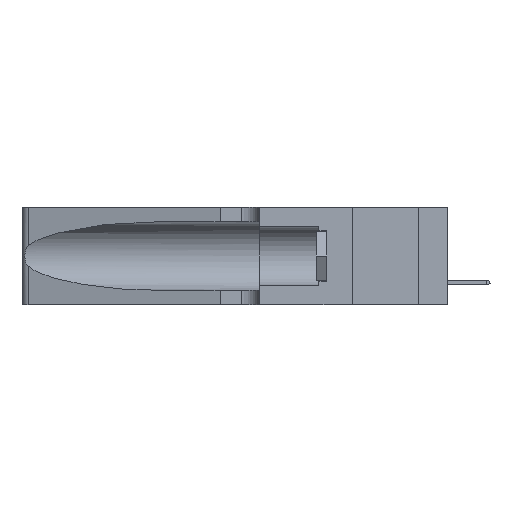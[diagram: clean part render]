
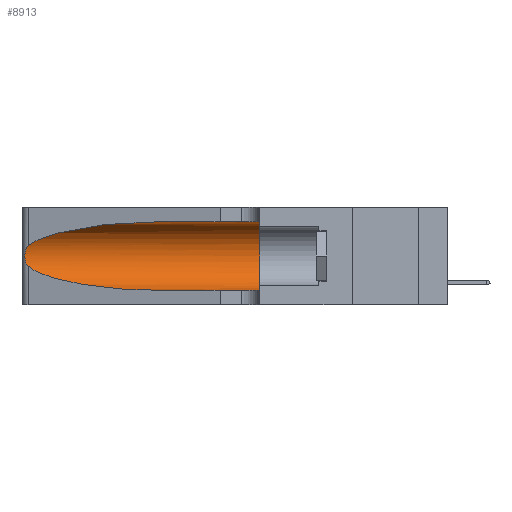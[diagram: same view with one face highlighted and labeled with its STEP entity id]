
A CAD part, left-side view. The second image highlights one B-rep face of the part: STEP entity #8913.
In plain terms, the highlighted cylindrical face has radius 3.308 mm (diameter 6.617 mm), a partial arc.
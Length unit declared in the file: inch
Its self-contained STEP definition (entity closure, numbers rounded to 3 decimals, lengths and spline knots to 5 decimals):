
#789 = CARTESIAN_POINT ( 'NONE',  ( 0.1305, 0.35, 0.05475 ) ) ;
#1953 = B_SPLINE_CURVE_WITH_KNOTS ( 'NONE', 3,
 ( #25652, #28455, #9611, #30937, #12276, #33630, #25879, #31040, #31159, #15073, #20415, #17869, #9949, #28571 ),
 .UNSPECIFIED., .F., .F.,
 ( 4, 2, 2, 2, 2, 2, 4 ),
 ( 0., 0.00027, 0.00053, 0.00107, 0.0016, 0.00187, 0.00214 ),
 .UNSPECIFIED. ) ;
#3556 = CARTESIAN_POINT ( 'NONE',  ( 0.18966, 0.96281, 0.05475 ) ) ;
#3749 = ORIENTED_EDGE ( 'NONE', *, *, #12329, .T. ) ;
#3765 = FACE_OUTER_BOUND ( 'NONE', #19042, .T. ) ;
#4085 = CIRCLE ( 'NONE', #7593, 0.13025 ) ;
#4809 = CARTESIAN_POINT ( 'NONE',  ( 0.2373, 1.15595, 0.28018 ) ) ;
#4878 = LINE ( 'NONE', #30529, #29453 ) ;
#5195 = DIRECTION ( 'NONE',  ( 0., -1., 0. ) ) ;
#5419 = EDGE_CURVE ( 'NONE', #30659, #13672, #1953, .T. ) ;
#6132 = CARTESIAN_POINT ( 'NONE',  ( 0.1305, 1.61858, 0.185 ) ) ;
#6133 = DIRECTION ( 'NONE',  ( 0., 1., 0. ) ) ;
#7593 = AXIS2_PLACEMENT_3D ( 'NONE', #32778, #6133, #11466 ) ;
#8037 = CARTESIAN_POINT ( 'NONE',  ( 0.1305, 0.72297, 0.05475 ) ) ;
#8913 = ADVANCED_FACE ( 'NONE', ( #3765 ), #20054, .F. ) ;
#9611 = CARTESIAN_POINT ( 'NONE',  ( 0.25639, 1.23184, 0.21858 ) ) ;
#9949 = CARTESIAN_POINT ( 'NONE',  ( 0.25555, 1.22993, 0.14849 ) ) ;
#11466 = DIRECTION ( 'NONE',  ( 0., 0., 1. ) ) ;
#11653 = CARTESIAN_POINT ( 'NONE',  ( 0.25487, 1.22718, 0.22369 ) ) ;
#12276 = CARTESIAN_POINT ( 'NONE',  ( 0.25854, 1.2359, 0.20912 ) ) ;
#12329 = EDGE_CURVE ( 'NONE', #13206, #30659, #30320, .T. ) ;
#13206 = VERTEX_POINT ( 'NONE', #31715 ) ;
#13304 = AXIS2_PLACEMENT_3D ( 'NONE', #6132, #24704, #30208 ) ;
#13672 = VERTEX_POINT ( 'NONE', #20605 ) ;
#13764 = ORIENTED_EDGE ( 'NONE', *, *, #5419, .T. ) ;
#14542 = VECTOR ( 'NONE', #5195, 39.37008 ) ;
#15073 = CARTESIAN_POINT ( 'NONE',  ( 0.25856, 1.23593, 0.16098 ) ) ;
#15747 = CARTESIAN_POINT ( 'NONE',  ( 0.25487, 1.22718, 0.22369 ) ) ;
#17377 = ORIENTED_EDGE ( 'NONE', *, *, #22622, .F. ) ;
#17453 = ORIENTED_EDGE ( 'NONE', *, *, #29007, .F. ) ;
#17869 = CARTESIAN_POINT ( 'NONE',  ( 0.25639, 1.23186, 0.15144 ) ) ;
#18022 = ORIENTED_EDGE ( 'NONE', *, *, #28373, .T. ) ;
#18400 = CARTESIAN_POINT ( 'NONE',  ( 0.18966, 0.96281, 0.31525 ) ) ;
#18597 = CARTESIAN_POINT ( 'NONE',  ( 0.2373, 1.15595, 0.08982 ) ) ;
#18759 = VERTEX_POINT ( 'NONE', #8037 ) ;
#19042 = EDGE_LOOP ( 'NONE', ( #3749, #13764, #18022, #25834, #17453, #17377 ) ) ;
#19198 = CARTESIAN_POINT ( 'NONE',  ( 0.25487, 1.22718, 0.14631 ) ) ;
#20054 = CYLINDRICAL_SURFACE ( 'NONE', #13304, 0.13025 ) ;
#20055 = DIRECTION ( 'NONE',  ( 0., -1., 0. ) ) ;
#20415 = CARTESIAN_POINT ( 'NONE',  ( 0.25789, 1.23486, 0.15765 ) ) ;
#20605 = CARTESIAN_POINT ( 'NONE',  ( 0.25487, 1.22718, 0.14631 ) ) ;
#20797 = LINE ( 'NONE', #21150, #14542 ) ;
#21150 = CARTESIAN_POINT ( 'NONE',  ( 0.1305, 1.61858, 0.31525 ) ) ;
#22183 = CARTESIAN_POINT ( 'NONE',  ( 0.1305, 0.72297, 0.05475 ) ) ;
#22622 = EDGE_CURVE ( 'NONE', #13206, #25965, #20797, .T. ) ;
#23707 =( BOUNDED_CURVE ( )  B_SPLINE_CURVE ( 3, ( #19198, #18597, #3556, #22183 ),
 .UNSPECIFIED., .F., .T. ) 
 B_SPLINE_CURVE_WITH_KNOTS ( ( 4, 4 ),
 ( 3.44316, 4.71239 ),
 .UNSPECIFIED. ) 
 CURVE ( )  GEOMETRIC_REPRESENTATION_ITEM ( )  RATIONAL_B_SPLINE_CURVE ( ( 1., 0.87, 0.87, 1. ) ) 
 REPRESENTATION_ITEM ( '' )  );
#24704 = DIRECTION ( 'NONE',  ( 0., -1., 0. ) ) ;
#25652 = CARTESIAN_POINT ( 'NONE',  ( 0.25487, 1.22718, 0.22369 ) ) ;
#25834 = ORIENTED_EDGE ( 'NONE', *, *, #29304, .T. ) ;
#25879 = CARTESIAN_POINT ( 'NONE',  ( 0.26075, 1.23896, 0.19203 ) ) ;
#25965 = VERTEX_POINT ( 'NONE', #26298 ) ;
#26298 = CARTESIAN_POINT ( 'NONE',  ( 0.1305, 0.35, 0.31525 ) ) ;
#28175 = VERTEX_POINT ( 'NONE', #789 ) ;
#28373 = EDGE_CURVE ( 'NONE', #13672, #18759, #23707, .T. ) ;
#28455 = CARTESIAN_POINT ( 'NONE',  ( 0.25555, 1.22994, 0.2215 ) ) ;
#28571 = CARTESIAN_POINT ( 'NONE',  ( 0.25487, 1.22718, 0.14631 ) ) ;
#29007 = EDGE_CURVE ( 'NONE', #25965, #28175, #4085, .T. ) ;
#29304 = EDGE_CURVE ( 'NONE', #18759, #28175, #4878, .T. ) ;
#29453 = VECTOR ( 'NONE', #20055, 39.37008 ) ;
#30208 = DIRECTION ( 'NONE',  ( 0., 0., -1. ) ) ;
#30320 =( BOUNDED_CURVE ( )  B_SPLINE_CURVE ( 3, ( #31262, #18400, #4809, #15747 ),
 .UNSPECIFIED., .F., .T. ) 
 B_SPLINE_CURVE_WITH_KNOTS ( ( 4, 4 ),
 ( 1.5708, 2.84003 ),
 .UNSPECIFIED. ) 
 CURVE ( )  GEOMETRIC_REPRESENTATION_ITEM ( )  RATIONAL_B_SPLINE_CURVE ( ( 1., 0.87, 0.87, 1. ) ) 
 REPRESENTATION_ITEM ( '' )  );
#30529 = CARTESIAN_POINT ( 'NONE',  ( 0.1305, 1.61858, 0.05475 ) ) ;
#30659 = VERTEX_POINT ( 'NONE', #11653 ) ;
#30937 = CARTESIAN_POINT ( 'NONE',  ( 0.25787, 1.23484, 0.2124 ) ) ;
#31040 = CARTESIAN_POINT ( 'NONE',  ( 0.26075, 1.23896, 0.178 ) ) ;
#31159 = CARTESIAN_POINT ( 'NONE',  ( 0.26017, 1.23833, 0.17102 ) ) ;
#31262 = CARTESIAN_POINT ( 'NONE',  ( 0.1305, 0.72297, 0.31525 ) ) ;
#31715 = CARTESIAN_POINT ( 'NONE',  ( 0.1305, 0.72297, 0.31525 ) ) ;
#32778 = CARTESIAN_POINT ( 'NONE',  ( 0.1305, 0.35, 0.185 ) ) ;
#33630 = CARTESIAN_POINT ( 'NONE',  ( 0.26018, 1.23835, 0.19895 ) ) ;
